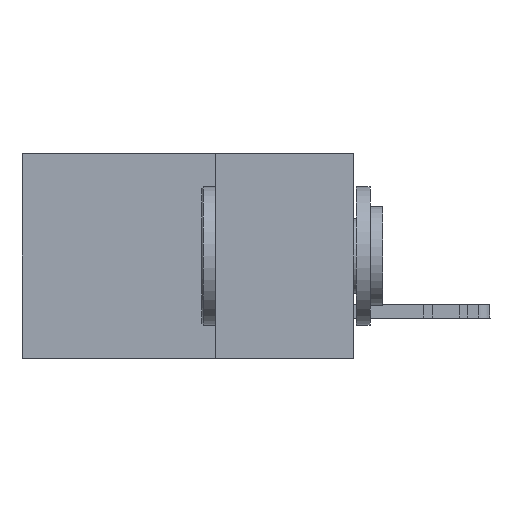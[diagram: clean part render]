
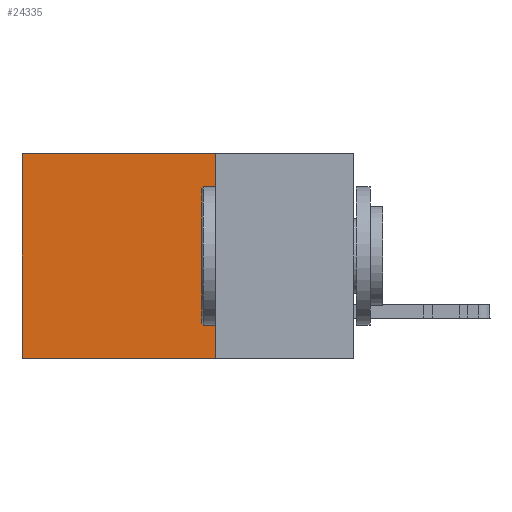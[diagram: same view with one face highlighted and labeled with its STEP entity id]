
A CAD part, left-side view. The second image highlights one B-rep face of the part: STEP entity #24335.
In plain terms, the highlighted planar face has unit normal (-1, 0, 0).
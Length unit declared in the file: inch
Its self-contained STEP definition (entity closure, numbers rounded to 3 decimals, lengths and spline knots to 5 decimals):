
#1078 = CARTESIAN_POINT ( 'NONE',  ( 0.2875, 0.25, 0. ) ) ;
#1454 = ORIENTED_EDGE ( 'NONE', *, *, #35456, .F. ) ;
#1495 = EDGE_CURVE ( 'NONE', #30214, #7418, #14670, .T. ) ;
#1578 = CARTESIAN_POINT ( 'NONE',  ( 0.2875, 0.6, -0.37 ) ) ;
#4145 = CARTESIAN_POINT ( 'NONE',  ( 0.2875, 0.25, 0. ) ) ;
#4737 = DIRECTION ( 'NONE',  ( 0., 0., -1. ) ) ;
#5184 = AXIS2_PLACEMENT_3D ( 'NONE', #4145, #38316, #4737 ) ;
#5849 = VERTEX_POINT ( 'NONE', #27565 ) ;
#6046 = LINE ( 'NONE', #18260, #26410 ) ;
#7418 = VERTEX_POINT ( 'NONE', #26497 ) ;
#14493 = DIRECTION ( 'NONE',  ( 0., 0., -1. ) ) ;
#14571 = VERTEX_POINT ( 'NONE', #1578 ) ;
#14670 = LINE ( 'NONE', #20791, #37236 ) ;
#17015 = VECTOR ( 'NONE', #25485, 39.37008 ) ;
#18229 = CARTESIAN_POINT ( 'NONE',  ( 0.2875, 0.25, 0. ) ) ;
#18260 = CARTESIAN_POINT ( 'NONE',  ( 0.2875, 0.25, -0.37 ) ) ;
#19805 = LINE ( 'NONE', #34664, #17015 ) ;
#20791 = CARTESIAN_POINT ( 'NONE',  ( 0.2875, 0.25, 0. ) ) ;
#21259 = DIRECTION ( 'NONE',  ( 0., 1., 0. ) ) ;
#21615 = EDGE_CURVE ( 'NONE', #30214, #5849, #27577, .T. ) ;
#23492 = EDGE_LOOP ( 'NONE', ( #29507, #1454, #38037, #28869 ) ) ;
#24335 = ADVANCED_FACE ( 'NONE', ( #38906 ), #35481, .F. ) ;
#25485 = DIRECTION ( 'NONE',  ( 0., 0., -1. ) ) ;
#26410 = VECTOR ( 'NONE', #27203, 39.37008 ) ;
#26497 = CARTESIAN_POINT ( 'NONE',  ( 0.2875, 0.25, -0.37 ) ) ;
#27203 = DIRECTION ( 'NONE',  ( 0., 1., 0. ) ) ;
#27565 = CARTESIAN_POINT ( 'NONE',  ( 0.2875, 0.6, 0. ) ) ;
#27577 = LINE ( 'NONE', #18229, #32762 ) ;
#28869 = ORIENTED_EDGE ( 'NONE', *, *, #21615, .T. ) ;
#29507 = ORIENTED_EDGE ( 'NONE', *, *, #30587, .T. ) ;
#30214 = VERTEX_POINT ( 'NONE', #1078 ) ;
#30587 = EDGE_CURVE ( 'NONE', #5849, #14571, #19805, .T. ) ;
#32762 = VECTOR ( 'NONE', #21259, 39.37008 ) ;
#34664 = CARTESIAN_POINT ( 'NONE',  ( 0.2875, 0.6, 0. ) ) ;
#35456 = EDGE_CURVE ( 'NONE', #7418, #14571, #6046, .T. ) ;
#35481 = PLANE ( 'NONE',  #5184 ) ;
#37236 = VECTOR ( 'NONE', #14493, 39.37008 ) ;
#38037 = ORIENTED_EDGE ( 'NONE', *, *, #1495, .F. ) ;
#38316 = DIRECTION ( 'NONE',  ( 1., 0., 0. ) ) ;
#38906 = FACE_OUTER_BOUND ( 'NONE', #23492, .T. ) ;
